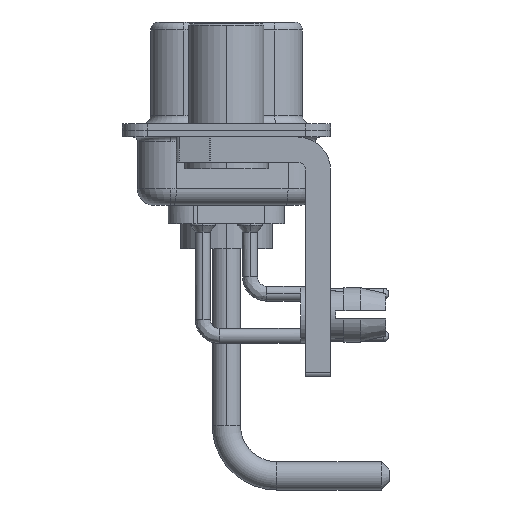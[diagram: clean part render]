
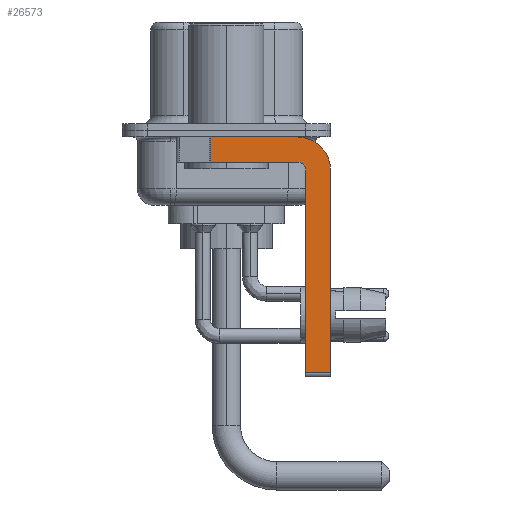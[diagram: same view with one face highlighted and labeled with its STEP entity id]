
A CAD part, left-side view. The second image highlights one B-rep face of the part: STEP entity #26573.
In plain terms, the highlighted planar face has unit normal (-1, 0, 0).
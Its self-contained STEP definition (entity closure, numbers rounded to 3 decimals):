
#429 = CARTESIAN_POINT ( 'NONE',  ( -2.9, -6.25, -2.4 ) ) ;
#1034 = CIRCLE ( 'NONE', #17998, 2. ) ;
#1191 = VERTEX_POINT ( 'NONE', #3772 ) ;
#2308 = LINE ( 'NONE', #11715, #3399 ) ;
#2505 = AXIS2_PLACEMENT_3D ( 'NONE', #26134, #14751, #7634 ) ;
#3051 = VERTEX_POINT ( 'NONE', #25871 ) ;
#3399 = VECTOR ( 'NONE', #20962, 1000. ) ;
#3772 = CARTESIAN_POINT ( 'NONE',  ( -2.9, -4.75, -14.55 ) ) ;
#4279 = ORIENTED_EDGE ( 'NONE', *, *, #22218, .F. ) ;
#4423 = CARTESIAN_POINT ( 'NONE',  ( -2.9, -4.25, -14.55 ) ) ;
#4574 = ORIENTED_EDGE ( 'NONE', *, *, #7074, .F. ) ;
#4611 = VECTOR ( 'NONE', #20439, 1000. ) ;
#5201 = ORIENTED_EDGE ( 'NONE', *, *, #5568, .F. ) ;
#5249 = ORIENTED_EDGE ( 'NONE', *, *, #26846, .F. ) ;
#5568 = EDGE_CURVE ( 'NONE', #18010, #7629, #25016, .T. ) ;
#5578 = AXIS2_PLACEMENT_3D ( 'NONE', #8565, #27067, #24636 ) ;
#6592 = ORIENTED_EDGE ( 'NONE', *, *, #24898, .T. ) ;
#7074 = EDGE_CURVE ( 'NONE', #27881, #3051, #17258, .T. ) ;
#7138 = CARTESIAN_POINT ( 'NONE',  ( -2.9, -4.25, -1.9 ) ) ;
#7584 = EDGE_CURVE ( 'NONE', #17974, #18010, #11902, .T. ) ;
#7629 = VERTEX_POINT ( 'NONE', #8119 ) ;
#7634 = DIRECTION ( 'NONE',  ( 0., 0., -1. ) ) ;
#8119 = CARTESIAN_POINT ( 'NONE',  ( -2.9, 0.978, -1.9 ) ) ;
#8545 = ORIENTED_EDGE ( 'NONE', *, *, #7584, .F. ) ;
#8565 = CARTESIAN_POINT ( 'NONE',  ( -2.9, -4.25, -2.4 ) ) ;
#9311 = CARTESIAN_POINT ( 'NONE',  ( -2.9, 0.978, -0.4 ) ) ;
#10344 = VERTEX_POINT ( 'NONE', #28531 ) ;
#11204 = CARTESIAN_POINT ( 'NONE',  ( -2.9, -4.25, -1.9 ) ) ;
#11715 = CARTESIAN_POINT ( 'NONE',  ( -2.9, 0.978, -1.9 ) ) ;
#11902 = CIRCLE ( 'NONE', #5578, 0.5 ) ;
#12691 = ORIENTED_EDGE ( 'NONE', *, *, #14449, .F. ) ;
#14124 = DIRECTION ( 'NONE',  ( 0., -1., 0. ) ) ;
#14449 = EDGE_CURVE ( 'NONE', #1191, #17974, #26452, .T. ) ;
#14751 = DIRECTION ( 'NONE',  ( 1., 0., 0. ) ) ;
#16579 = PLANE ( 'NONE',  #2505 ) ;
#16672 = CARTESIAN_POINT ( 'NONE',  ( -2.9, 3., -0.4 ) ) ;
#17258 = LINE ( 'NONE', #16672, #29810 ) ;
#17974 = VERTEX_POINT ( 'NONE', #23081 ) ;
#17998 = AXIS2_PLACEMENT_3D ( 'NONE', #26439, #19733, #20036 ) ;
#18003 = VECTOR ( 'NONE', #25936, 1000. ) ;
#18010 = VERTEX_POINT ( 'NONE', #7138 ) ;
#19607 = CARTESIAN_POINT ( 'NONE',  ( -2.9, -4.75, -14.8 ) ) ;
#19733 = DIRECTION ( 'NONE',  ( 1., 0., 0. ) ) ;
#20036 = DIRECTION ( 'NONE',  ( 0., 0., -1. ) ) ;
#20338 = VECTOR ( 'NONE', #28873, 1000. ) ;
#20439 = DIRECTION ( 'NONE',  ( 0., 1., 0. ) ) ;
#20796 = EDGE_CURVE ( 'NONE', #27881, #7629, #2308, .T. ) ;
#20854 = VERTEX_POINT ( 'NONE', #28677 ) ;
#20962 = DIRECTION ( 'NONE',  ( 0., 0., -1. ) ) ;
#20965 = LINE ( 'NONE', #4423, #26318 ) ;
#21437 = FACE_OUTER_BOUND ( 'NONE', #26895, .T. ) ;
#22218 = EDGE_CURVE ( 'NONE', #10344, #20854, #28357, .T. ) ;
#22389 = ORIENTED_EDGE ( 'NONE', *, *, #20796, .T. ) ;
#22401 = DIRECTION ( 'NONE',  ( 0., -1., 0. ) ) ;
#23081 = CARTESIAN_POINT ( 'NONE',  ( -2.9, -4.75, -2.4 ) ) ;
#24636 = DIRECTION ( 'NONE',  ( 0., 0., 1. ) ) ;
#24898 = EDGE_CURVE ( 'NONE', #1191, #20854, #20965, .T. ) ;
#25016 = LINE ( 'NONE', #11204, #4611 ) ;
#25871 = CARTESIAN_POINT ( 'NONE',  ( -2.9, -4.25, -0.4 ) ) ;
#25936 = DIRECTION ( 'NONE',  ( 0., 0., -1. ) ) ;
#26134 = CARTESIAN_POINT ( 'NONE',  ( -2.9, -4.25, -2.4 ) ) ;
#26318 = VECTOR ( 'NONE', #14124, 1000. ) ;
#26439 = CARTESIAN_POINT ( 'NONE',  ( -2.9, -4.25, -2.4 ) ) ;
#26452 = LINE ( 'NONE', #19607, #20338 ) ;
#26573 = ADVANCED_FACE ( 'NONE', ( #21437 ), #16579, .F. ) ;
#26846 = EDGE_CURVE ( 'NONE', #3051, #10344, #1034, .T. ) ;
#26895 = EDGE_LOOP ( 'NONE', ( #4574, #22389, #5201, #8545, #12691, #6592, #4279, #5249 ) ) ;
#27067 = DIRECTION ( 'NONE',  ( -1., 0., 0. ) ) ;
#27881 = VERTEX_POINT ( 'NONE', #9311 ) ;
#28357 = LINE ( 'NONE', #429, #18003 ) ;
#28531 = CARTESIAN_POINT ( 'NONE',  ( -2.9, -6.25, -2.4 ) ) ;
#28677 = CARTESIAN_POINT ( 'NONE',  ( -2.9, -6.25, -14.55 ) ) ;
#28873 = DIRECTION ( 'NONE',  ( 0., 0., 1. ) ) ;
#29810 = VECTOR ( 'NONE', #22401, 1000. ) ;
